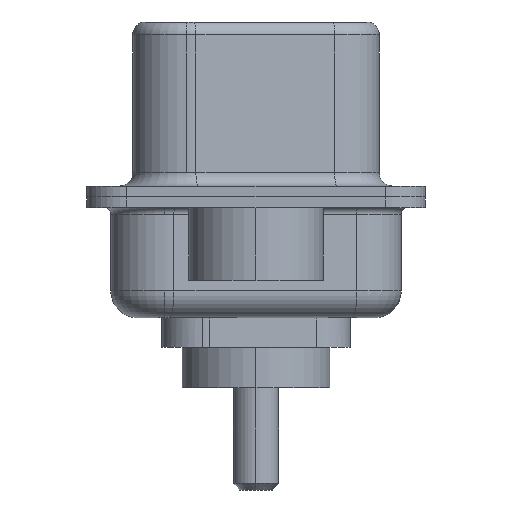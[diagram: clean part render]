
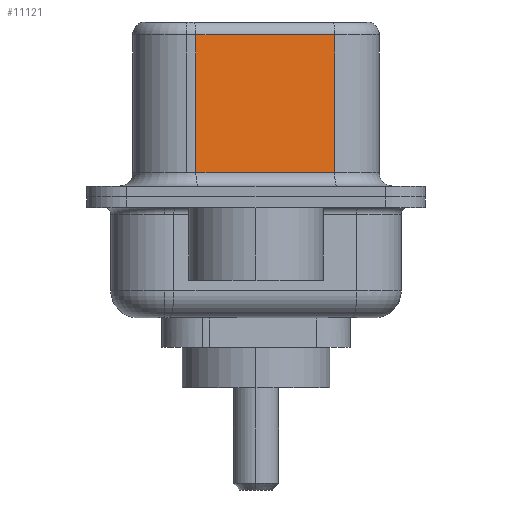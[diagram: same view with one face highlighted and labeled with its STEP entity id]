
A CAD part, left-side view. The second image highlights one B-rep face of the part: STEP entity #11121.
In plain terms, the highlighted planar face has unit normal (-0.985, -0.174, 0).
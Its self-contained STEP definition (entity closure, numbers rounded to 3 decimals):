
#99 = ORIENTED_EDGE ( 'NONE', *, *, #9659, .T. ) ;
#109 = EDGE_CURVE ( 'NONE', #5558, #574, #10381, .T. ) ;
#574 = VERTEX_POINT ( 'NONE', #1683 ) ;
#862 = CARTESIAN_POINT ( 'NONE',  ( 4.565, -2.927, 6.02 ) ) ;
#1259 = EDGE_CURVE ( 'NONE', #7006, #1986, #5169, .T. ) ;
#1471 = ORIENTED_EDGE ( 'NONE', *, *, #9859, .T. ) ;
#1641 = FACE_OUTER_BOUND ( 'NONE', #2606, .T. ) ;
#1683 = CARTESIAN_POINT ( 'NONE',  ( 4.565, -2.927, 0.9 ) ) ;
#1986 = VERTEX_POINT ( 'NONE', #4864 ) ;
#2606 = EDGE_LOOP ( 'NONE', ( #8000, #1471, #12678, #99 ) ) ;
#3023 = DIRECTION ( 'NONE',  ( 0.174, -0.985, 0. ) ) ;
#3368 = CARTESIAN_POINT ( 'NONE',  ( 4.565, -2.927, 6.52 ) ) ;
#4326 = CARTESIAN_POINT ( 'NONE',  ( 4.565, -2.927, 6.02 ) ) ;
#4751 = CARTESIAN_POINT ( 'NONE',  ( 3.655, 2.233, 6.52 ) ) ;
#4812 = CARTESIAN_POINT ( 'NONE',  ( 4.565, -2.927, 6.52 ) ) ;
#4864 = CARTESIAN_POINT ( 'NONE',  ( 3.655, 2.233, 0.9 ) ) ;
#4959 = DIRECTION ( 'NONE',  ( 0., 0., -1. ) ) ;
#5055 = DIRECTION ( 'NONE',  ( 0., 0., -1. ) ) ;
#5169 = LINE ( 'NONE', #4751, #12302 ) ;
#5186 = VECTOR ( 'NONE', #5055, 1000. ) ;
#5488 = DIRECTION ( 'NONE',  ( 0.985, 0.174, 0. ) ) ;
#5558 = VERTEX_POINT ( 'NONE', #862 ) ;
#7006 = VERTEX_POINT ( 'NONE', #9244 ) ;
#8000 = ORIENTED_EDGE ( 'NONE', *, *, #109, .F. ) ;
#8479 = LINE ( 'NONE', #4326, #10989 ) ;
#9244 = CARTESIAN_POINT ( 'NONE',  ( 3.655, 2.233, 6.02 ) ) ;
#9386 = PLANE ( 'NONE',  #11547 ) ;
#9659 = EDGE_CURVE ( 'NONE', #1986, #574, #10848, .T. ) ;
#9859 = EDGE_CURVE ( 'NONE', #5558, #7006, #8479, .T. ) ;
#9970 = CARTESIAN_POINT ( 'NONE',  ( 4.565, -2.927, 0.9 ) ) ;
#10259 = DIRECTION ( 'NONE',  ( -0.174, 0.985, 0. ) ) ;
#10381 = LINE ( 'NONE', #4812, #5186 ) ;
#10555 = VECTOR ( 'NONE', #3023, 1000. ) ;
#10848 = LINE ( 'NONE', #9970, #10555 ) ;
#10989 = VECTOR ( 'NONE', #10259, 1000. ) ;
#11121 = ADVANCED_FACE ( 'NONE', ( #1641 ), #9386, .F. ) ;
#11547 = AXIS2_PLACEMENT_3D ( 'NONE', #3368, #5488, #12233 ) ;
#12233 = DIRECTION ( 'NONE',  ( -0.174, 0.985, 0. ) ) ;
#12302 = VECTOR ( 'NONE', #4959, 1000. ) ;
#12678 = ORIENTED_EDGE ( 'NONE', *, *, #1259, .T. ) ;
